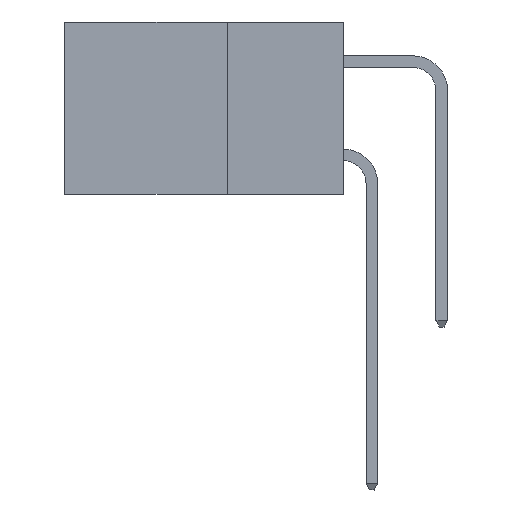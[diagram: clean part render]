
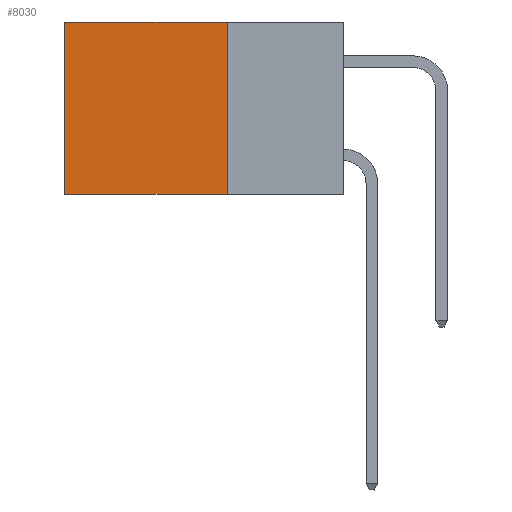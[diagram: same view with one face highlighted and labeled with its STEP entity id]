
A CAD part, left-side view. The second image highlights one B-rep face of the part: STEP entity #8030.
In plain terms, the highlighted planar face has unit normal (-1, 0, 0).
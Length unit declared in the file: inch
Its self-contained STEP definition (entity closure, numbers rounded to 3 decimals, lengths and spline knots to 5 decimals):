
#803 = CARTESIAN_POINT ( 'NONE',  ( 0.2615, 0.6, -0.37 ) ) ;
#1242 = DIRECTION ( 'NONE',  ( 0., 1., 0. ) ) ;
#1455 = ORIENTED_EDGE ( 'NONE', *, *, #3294, .F. ) ;
#1500 = VERTEX_POINT ( 'NONE', #15871 ) ;
#2471 = VERTEX_POINT ( 'NONE', #6828 ) ;
#2684 = EDGE_CURVE ( 'NONE', #10744, #1500, #11826, .T. ) ;
#3294 = EDGE_CURVE ( 'NONE', #1500, #7835, #9606, .T. ) ;
#3491 = CARTESIAN_POINT ( 'NONE',  ( 0.2615, 0.25, -0.37 ) ) ;
#4064 = FACE_OUTER_BOUND ( 'NONE', #11408, .T. ) ;
#4405 = CARTESIAN_POINT ( 'NONE',  ( 0.2615, 0.25, -0.37 ) ) ;
#5206 = VECTOR ( 'NONE', #14366, 39.37008 ) ;
#6036 = AXIS2_PLACEMENT_3D ( 'NONE', #8876, #9036, #11327 ) ;
#6828 = CARTESIAN_POINT ( 'NONE',  ( 0.2615, 0.6, 0. ) ) ;
#7014 = LINE ( 'NONE', #13052, #13319 ) ;
#7835 = VERTEX_POINT ( 'NONE', #803 ) ;
#8030 = ADVANCED_FACE ( 'NONE', ( #4064 ), #12395, .F. ) ;
#8335 = DIRECTION ( 'NONE',  ( 0., 0., -1. ) ) ;
#8581 = EDGE_CURVE ( 'NONE', #2471, #7835, #7014, .T. ) ;
#8756 = CARTESIAN_POINT ( 'NONE',  ( 0.2615, 0.25, 0. ) ) ;
#8784 = EDGE_CURVE ( 'NONE', #10744, #2471, #12082, .T. ) ;
#8812 = CARTESIAN_POINT ( 'NONE',  ( 0.2615, 0.25, 0. ) ) ;
#8876 = CARTESIAN_POINT ( 'NONE',  ( 0.2615, 0.25, -0.37 ) ) ;
#9036 = DIRECTION ( 'NONE',  ( 1., 0., 0. ) ) ;
#9606 = LINE ( 'NONE', #3491, #14849 ) ;
#10744 = VERTEX_POINT ( 'NONE', #8812 ) ;
#11150 = ORIENTED_EDGE ( 'NONE', *, *, #2684, .F. ) ;
#11327 = DIRECTION ( 'NONE',  ( 0., 0., -1. ) ) ;
#11408 = EDGE_LOOP ( 'NONE', ( #14166, #1455, #11150, #14296 ) ) ;
#11826 = LINE ( 'NONE', #4405, #5206 ) ;
#12045 = DIRECTION ( 'NONE',  ( 0., 1., 0. ) ) ;
#12082 = LINE ( 'NONE', #8756, #14662 ) ;
#12395 = PLANE ( 'NONE',  #6036 ) ;
#13052 = CARTESIAN_POINT ( 'NONE',  ( 0.2615, 0.6, -0.37 ) ) ;
#13319 = VECTOR ( 'NONE', #8335, 39.37008 ) ;
#14166 = ORIENTED_EDGE ( 'NONE', *, *, #8581, .T. ) ;
#14296 = ORIENTED_EDGE ( 'NONE', *, *, #8784, .T. ) ;
#14366 = DIRECTION ( 'NONE',  ( 0., 0., -1. ) ) ;
#14662 = VECTOR ( 'NONE', #1242, 39.37008 ) ;
#14849 = VECTOR ( 'NONE', #12045, 39.37008 ) ;
#15871 = CARTESIAN_POINT ( 'NONE',  ( 0.2615, 0.25, -0.37 ) ) ;
